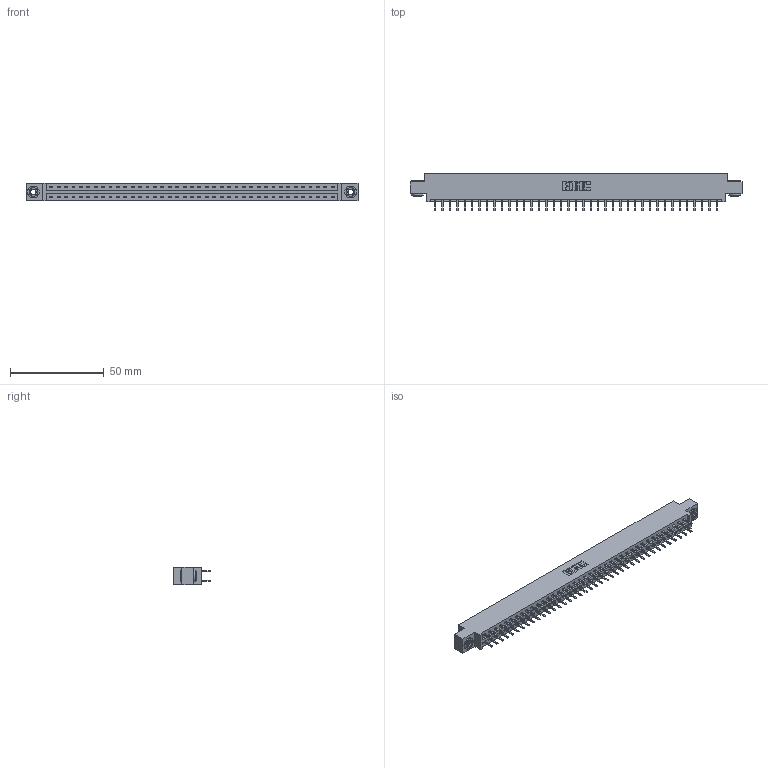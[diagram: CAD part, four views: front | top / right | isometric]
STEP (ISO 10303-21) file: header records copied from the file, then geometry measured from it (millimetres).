
FILE_DESCRIPTION (( 'STEP AP203' ), '1' );
FILE_NAME ('387-078-520-803.STEP', '2018-09-23T16:35:02', ( '' ), ( '' ), 'SwSTEP 2.0', 'SolidWorks 2016', '' );
FILE_SCHEMA (( 'CONFIG_CONTROL_DESIGN' ));
Length unit declared in the file: inch
Products named in the file (4): 337 Part_0.170 Offset - 0.156 Dia-TH; 345-292-001_345-293-120; 345-250-002_345-250-002-102; 387-078-520-803
Assembly tree (81 placements, depth 2):
  387-078-520-803
    337 Part_0.170 Offset - 0.156 Dia-TH
    345-292-001_345-293-120  x78
    345-250-002_345-250-002-102  x2
Bounding box: 177.55 x 20.02 x 9.4 mm (x, y, z)
Volume: 18538.9 mm3; surface area: 21163.5 mm2
Topology: 81 solids, 81 shells, 4680 faces, 13581 edges, 8842 vertices
Faces by surface type: plane 3204, cylinder 1468, cone 8
Entity records: 31522 total; most frequent: CARTESIAN_POINT 5301, ORIENTED_EDGE 5218, DIRECTION 4535, EDGE_CURVE 2609, LINE 2453, VECTOR 2453, VERTEX_POINT 1734, AXIS2_PLACEMENT_3D 1041
